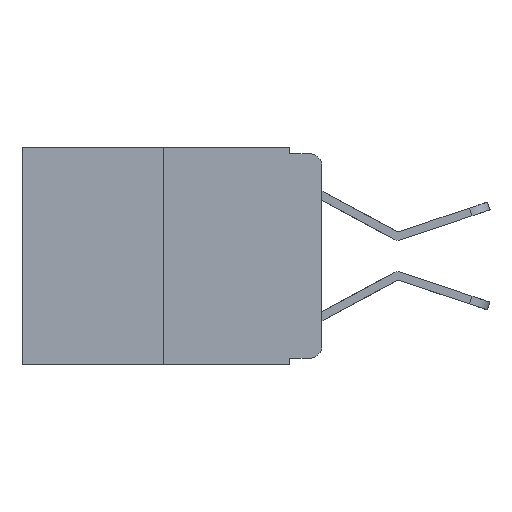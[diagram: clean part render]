
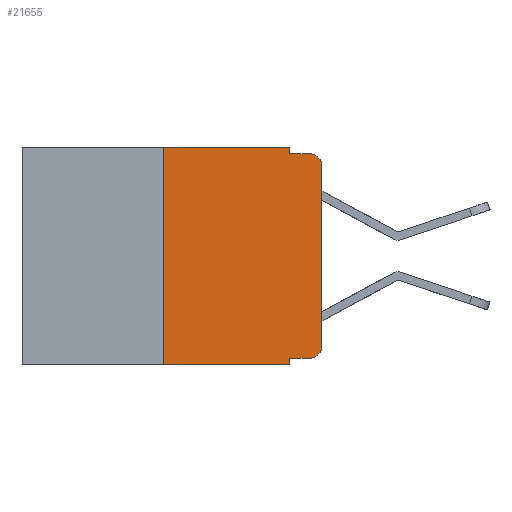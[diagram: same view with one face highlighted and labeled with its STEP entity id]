
A CAD part, left-side view. The second image highlights one B-rep face of the part: STEP entity #21655.
In plain terms, the highlighted planar face has unit normal (-1, 0, 0).
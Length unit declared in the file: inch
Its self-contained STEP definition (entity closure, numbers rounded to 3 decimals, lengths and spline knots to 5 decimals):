
#538 = LINE ( 'NONE', #5673, #14646 ) ;
#1516 = DIRECTION ( 'NONE',  ( 0., 0., -1. ) ) ;
#1553 = DIRECTION ( 'NONE',  ( 0., 0., -1. ) ) ;
#1642 = EDGE_CURVE ( 'NONE', #15301, #7596, #11638, .T. ) ;
#1799 = VECTOR ( 'NONE', #10332, 39.37008 ) ;
#1860 = EDGE_LOOP ( 'NONE', ( #23203, #22135, #4396, #6763, #23164, #16126, #10783, #20784, #3404, #21988 ) ) ;
#2754 = EDGE_CURVE ( 'NONE', #18987, #12507, #13297, .T. ) ;
#3202 = CARTESIAN_POINT ( 'NONE',  ( 0., 0.02, -0.333 ) ) ;
#3322 = CARTESIAN_POINT ( 'NONE',  ( 0., 0.051, 0. ) ) ;
#3328 = CIRCLE ( 'NONE', #14818, 0.02 ) ;
#3404 = ORIENTED_EDGE ( 'NONE', *, *, #12030, .T. ) ;
#3535 = VERTEX_POINT ( 'NONE', #3322 ) ;
#3592 = EDGE_CURVE ( 'NONE', #7138, #12507, #5230, .T. ) ;
#4054 = VECTOR ( 'NONE', #1516, 39.37008 ) ;
#4226 = EDGE_CURVE ( 'NONE', #16615, #3535, #538, .T. ) ;
#4396 = ORIENTED_EDGE ( 'NONE', *, *, #20295, .F. ) ;
#4803 = CARTESIAN_POINT ( 'NONE',  ( 0., 0.051, -0.01 ) ) ;
#4904 = VERTEX_POINT ( 'NONE', #7496 ) ;
#5053 = CARTESIAN_POINT ( 'NONE',  ( 0., 0., -0.03 ) ) ;
#5230 = LINE ( 'NONE', #12418, #4054 ) ;
#5368 = DIRECTION ( 'NONE',  ( 0., -1., 0. ) ) ;
#5673 = CARTESIAN_POINT ( 'NONE',  ( 0., 0.473, 0. ) ) ;
#5876 = EDGE_CURVE ( 'NONE', #22249, #15301, #19006, .T. ) ;
#6589 = EDGE_CURVE ( 'NONE', #3535, #11875, #23235, .T. ) ;
#6722 = CARTESIAN_POINT ( 'NONE',  ( 0., 0.25, 0. ) ) ;
#6763 = ORIENTED_EDGE ( 'NONE', *, *, #6589, .F. ) ;
#6792 = LINE ( 'NONE', #14484, #14752 ) ;
#7013 = DIRECTION ( 'NONE',  ( 1., 0., 0. ) ) ;
#7138 = VERTEX_POINT ( 'NONE', #21734 ) ;
#7496 = CARTESIAN_POINT ( 'NONE',  ( 0., 0.02, -0.01 ) ) ;
#7596 = VERTEX_POINT ( 'NONE', #5053 ) ;
#7936 = DIRECTION ( 'NONE',  ( 0., 0., 1. ) ) ;
#8137 = DIRECTION ( 'NONE',  ( 0., -1., 0. ) ) ;
#8960 = CARTESIAN_POINT ( 'NONE',  ( 0., 0.02, -0.313 ) ) ;
#9301 = EDGE_CURVE ( 'NONE', #18987, #16615, #15693, .T. ) ;
#9698 = EDGE_CURVE ( 'NONE', #7596, #4904, #3328, .T. ) ;
#10323 = FACE_OUTER_BOUND ( 'NONE', #1860, .T. ) ;
#10332 = DIRECTION ( 'NONE',  ( 0., 0., 1. ) ) ;
#10783 = ORIENTED_EDGE ( 'NONE', *, *, #2754, .T. ) ;
#10791 = DIRECTION ( 'NONE',  ( 0., 0., -1. ) ) ;
#11257 = AXIS2_PLACEMENT_3D ( 'NONE', #17841, #7013, #19593 ) ;
#11638 = LINE ( 'NONE', #18699, #1799 ) ;
#11875 = VERTEX_POINT ( 'NONE', #4803 ) ;
#12030 = EDGE_CURVE ( 'NONE', #7138, #22249, #6792, .T. ) ;
#12075 = LINE ( 'NONE', #20638, #17956 ) ;
#12418 = CARTESIAN_POINT ( 'NONE',  ( 0., 0.051, 0. ) ) ;
#12507 = VERTEX_POINT ( 'NONE', #12564 ) ;
#12564 = CARTESIAN_POINT ( 'NONE',  ( 0., 0.051, -0.343 ) ) ;
#12595 = DIRECTION ( 'NONE',  ( -1., 0., 0. ) ) ;
#12716 = DIRECTION ( 'NONE',  ( 0., 0., -1. ) ) ;
#12743 = VECTOR ( 'NONE', #17049, 39.37008 ) ;
#13297 = LINE ( 'NONE', #18006, #12743 ) ;
#14484 = CARTESIAN_POINT ( 'NONE',  ( 0., 0.051, -0.333 ) ) ;
#14578 = DIRECTION ( 'NONE',  ( 0., -1., 0. ) ) ;
#14646 = VECTOR ( 'NONE', #14578, 39.37008 ) ;
#14752 = VECTOR ( 'NONE', #5368, 39.37008 ) ;
#14818 = AXIS2_PLACEMENT_3D ( 'NONE', #23092, #12595, #1553 ) ;
#15301 = VERTEX_POINT ( 'NONE', #21059 ) ;
#15693 = LINE ( 'NONE', #18698, #16265 ) ;
#16070 = PLANE ( 'NONE',  #11257 ) ;
#16126 = ORIENTED_EDGE ( 'NONE', *, *, #9301, .F. ) ;
#16265 = VECTOR ( 'NONE', #7936, 39.37008 ) ;
#16615 = VERTEX_POINT ( 'NONE', #6722 ) ;
#17049 = DIRECTION ( 'NONE',  ( 0., -1., 0. ) ) ;
#17841 = CARTESIAN_POINT ( 'NONE',  ( 0., 0.473, 0. ) ) ;
#17956 = VECTOR ( 'NONE', #8137, 39.37008 ) ;
#18006 = CARTESIAN_POINT ( 'NONE',  ( 0., 0.473, -0.343 ) ) ;
#18698 = CARTESIAN_POINT ( 'NONE',  ( 0., 0.25, 0. ) ) ;
#18699 = CARTESIAN_POINT ( 'NONE',  ( 0., 0., 0. ) ) ;
#18987 = VERTEX_POINT ( 'NONE', #21826 ) ;
#19006 = CIRCLE ( 'NONE', #21307, 0.02 ) ;
#19593 = DIRECTION ( 'NONE',  ( 0., 0., -1. ) ) ;
#20295 = EDGE_CURVE ( 'NONE', #11875, #4904, #12075, .T. ) ;
#20638 = CARTESIAN_POINT ( 'NONE',  ( 0., 0.051, -0.01 ) ) ;
#20784 = ORIENTED_EDGE ( 'NONE', *, *, #3592, .F. ) ;
#21059 = CARTESIAN_POINT ( 'NONE',  ( 0., 0., -0.313 ) ) ;
#21307 = AXIS2_PLACEMENT_3D ( 'NONE', #8960, #21409, #10791 ) ;
#21409 = DIRECTION ( 'NONE',  ( -1., 0., 0. ) ) ;
#21655 = ADVANCED_FACE ( 'NONE', ( #10323 ), #16070, .F. ) ;
#21734 = CARTESIAN_POINT ( 'NONE',  ( 0., 0.051, -0.333 ) ) ;
#21826 = CARTESIAN_POINT ( 'NONE',  ( 0., 0.25, -0.343 ) ) ;
#21988 = ORIENTED_EDGE ( 'NONE', *, *, #5876, .T. ) ;
#22135 = ORIENTED_EDGE ( 'NONE', *, *, #9698, .T. ) ;
#22249 = VERTEX_POINT ( 'NONE', #3202 ) ;
#22725 = VECTOR ( 'NONE', #12716, 39.37008 ) ;
#23092 = CARTESIAN_POINT ( 'NONE',  ( 0., 0.02, -0.03 ) ) ;
#23164 = ORIENTED_EDGE ( 'NONE', *, *, #4226, .F. ) ;
#23197 = CARTESIAN_POINT ( 'NONE',  ( 0., 0.051, 0. ) ) ;
#23203 = ORIENTED_EDGE ( 'NONE', *, *, #1642, .T. ) ;
#23235 = LINE ( 'NONE', #23197, #22725 ) ;
